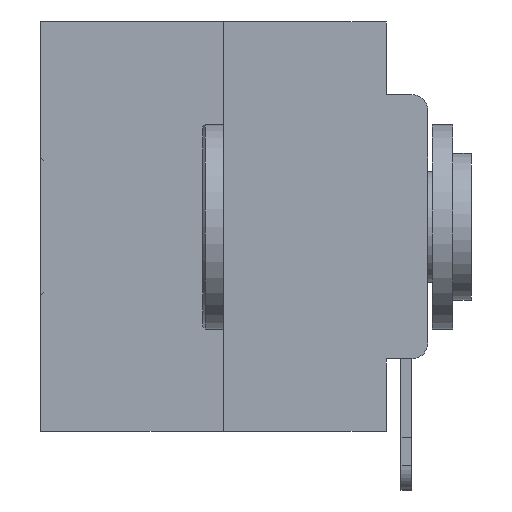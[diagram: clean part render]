
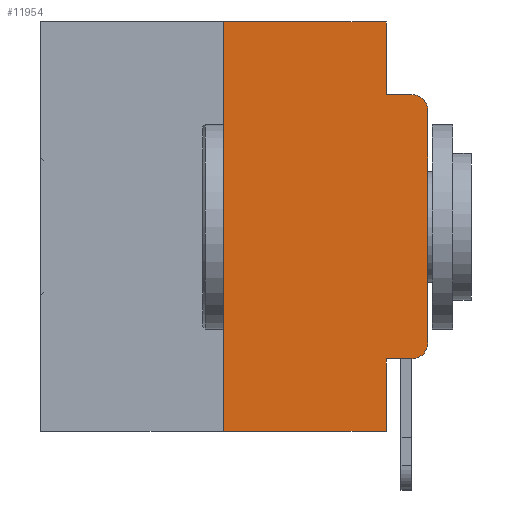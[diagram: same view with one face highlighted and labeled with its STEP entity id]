
A CAD part, left-side view. The second image highlights one B-rep face of the part: STEP entity #11954.
In plain terms, the highlighted planar face has unit normal (-1, 0, 0).
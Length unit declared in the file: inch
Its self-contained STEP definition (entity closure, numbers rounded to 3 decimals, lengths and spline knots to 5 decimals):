
#270 = VERTEX_POINT ( 'NONE', #3833 ) ;
#324 = VECTOR ( 'NONE', #23057, 39.37008 ) ;
#1065 = ORIENTED_EDGE ( 'NONE', *, *, #15553, .F. ) ;
#1364 = VERTEX_POINT ( 'NONE', #24609 ) ;
#1551 = DIRECTION ( 'NONE',  ( 0., -1., 0. ) ) ;
#1678 = CARTESIAN_POINT ( 'NONE',  ( 0., 0.051, -0.4115 ) ) ;
#2303 = VERTEX_POINT ( 'NONE', #25746 ) ;
#2864 = DIRECTION ( 'NONE',  ( -1., 0., 0. ) ) ;
#3169 = ORIENTED_EDGE ( 'NONE', *, *, #7215, .T. ) ;
#3351 = CARTESIAN_POINT ( 'NONE',  ( 0., 0.051, -0.0885 ) ) ;
#3833 = CARTESIAN_POINT ( 'NONE',  ( 0., 0.051, -0.4115 ) ) ;
#3913 = CARTESIAN_POINT ( 'NONE',  ( 0., 0., -0.3915 ) ) ;
#4246 = LINE ( 'NONE', #1678, #11834 ) ;
#4282 = CARTESIAN_POINT ( 'NONE',  ( 0., 0.473, -0.5 ) ) ;
#4827 = DIRECTION ( 'NONE',  ( 0., 0., -1. ) ) ;
#4832 = VECTOR ( 'NONE', #1551, 39.37008 ) ;
#7215 = EDGE_CURVE ( 'NONE', #31424, #12259, #27190, .T. ) ;
#8551 = EDGE_CURVE ( 'NONE', #28924, #19946, #29619, .T. ) ;
#8594 = VECTOR ( 'NONE', #22149, 39.37008 ) ;
#8623 = CARTESIAN_POINT ( 'NONE',  ( 0., 0., -0.1085 ) ) ;
#9428 = LINE ( 'NONE', #31160, #8594 ) ;
#9579 = CARTESIAN_POINT ( 'NONE',  ( 0., 0.02, -0.3915 ) ) ;
#11570 = ORIENTED_EDGE ( 'NONE', *, *, #25066, .F. ) ;
#11834 = VECTOR ( 'NONE', #19168, 39.37008 ) ;
#11904 = VECTOR ( 'NONE', #29697, 39.37008 ) ;
#11954 = ADVANCED_FACE ( 'NONE', ( #16748 ), #31044, .F. ) ;
#12088 = DIRECTION ( 'NONE',  ( 0., 0., -1. ) ) ;
#12253 = VERTEX_POINT ( 'NONE', #23450 ) ;
#12259 = VERTEX_POINT ( 'NONE', #3913 ) ;
#12339 = EDGE_CURVE ( 'NONE', #270, #31424, #4246, .T. ) ;
#12411 = DIRECTION ( 'NONE',  ( 0., 0., -1. ) ) ;
#13102 = CIRCLE ( 'NONE', #13474, 0.02 ) ;
#13474 = AXIS2_PLACEMENT_3D ( 'NONE', #17809, #2864, #20239 ) ;
#15224 = CARTESIAN_POINT ( 'NONE',  ( 0., 0.25, -0.5 ) ) ;
#15553 = EDGE_CURVE ( 'NONE', #270, #12253, #21610, .T. ) ;
#15741 = CARTESIAN_POINT ( 'NONE',  ( 0., 0., 0. ) ) ;
#15785 = EDGE_LOOP ( 'NONE', ( #17207, #23565, #11570, #17952, #18705, #24981, #20217, #1065, #21745, #3169 ) ) ;
#16651 = CARTESIAN_POINT ( 'NONE',  ( 0., 0.473, 0. ) ) ;
#16748 = FACE_OUTER_BOUND ( 'NONE', #15785, .T. ) ;
#17147 = EDGE_CURVE ( 'NONE', #26517, #28924, #9428, .T. ) ;
#17187 = CARTESIAN_POINT ( 'NONE',  ( 0., 0.473, 0. ) ) ;
#17207 = ORIENTED_EDGE ( 'NONE', *, *, #31098, .T. ) ;
#17559 = EDGE_CURVE ( 'NONE', #26517, #12253, #26884, .T. ) ;
#17809 = CARTESIAN_POINT ( 'NONE',  ( 0., 0.02, -0.1085 ) ) ;
#17952 = ORIENTED_EDGE ( 'NONE', *, *, #21983, .F. ) ;
#18024 = VERTEX_POINT ( 'NONE', #8623 ) ;
#18705 = ORIENTED_EDGE ( 'NONE', *, *, #8551, .F. ) ;
#19105 = DIRECTION ( 'NONE',  ( 0., -1., 0. ) ) ;
#19168 = DIRECTION ( 'NONE',  ( 0., -1., 0. ) ) ;
#19599 = DIRECTION ( 'NONE',  ( 1., 0., 0. ) ) ;
#19946 = VERTEX_POINT ( 'NONE', #25311 ) ;
#20047 = DIRECTION ( 'NONE',  ( 0., 0., -1. ) ) ;
#20217 = ORIENTED_EDGE ( 'NONE', *, *, #17559, .T. ) ;
#20239 = DIRECTION ( 'NONE',  ( 0., 0., -1. ) ) ;
#20328 = LINE ( 'NONE', #3351, #324 ) ;
#20421 = LINE ( 'NONE', #22462, #25844 ) ;
#21490 = CARTESIAN_POINT ( 'NONE',  ( 0., 0.02, -0.4115 ) ) ;
#21610 = LINE ( 'NONE', #26538, #27677 ) ;
#21745 = ORIENTED_EDGE ( 'NONE', *, *, #12339, .T. ) ;
#21983 = EDGE_CURVE ( 'NONE', #19946, #2303, #20421, .T. ) ;
#22149 = DIRECTION ( 'NONE',  ( 0., 0., 1. ) ) ;
#22462 = CARTESIAN_POINT ( 'NONE',  ( 0., 0.051, 0. ) ) ;
#23057 = DIRECTION ( 'NONE',  ( 0., -1., 0. ) ) ;
#23450 = CARTESIAN_POINT ( 'NONE',  ( 0., 0.051, -0.5 ) ) ;
#23565 = ORIENTED_EDGE ( 'NONE', *, *, #26559, .T. ) ;
#23865 = AXIS2_PLACEMENT_3D ( 'NONE', #9579, #26249, #12088 ) ;
#24589 = LINE ( 'NONE', #15741, #11904 ) ;
#24609 = CARTESIAN_POINT ( 'NONE',  ( 0., 0.02, -0.0885 ) ) ;
#24981 = ORIENTED_EDGE ( 'NONE', *, *, #17147, .F. ) ;
#25066 = EDGE_CURVE ( 'NONE', #2303, #1364, #20328, .T. ) ;
#25311 = CARTESIAN_POINT ( 'NONE',  ( 0., 0.051, 0. ) ) ;
#25746 = CARTESIAN_POINT ( 'NONE',  ( 0., 0.051, -0.0885 ) ) ;
#25844 = VECTOR ( 'NONE', #20047, 39.37008 ) ;
#26249 = DIRECTION ( 'NONE',  ( -1., 0., 0. ) ) ;
#26517 = VERTEX_POINT ( 'NONE', #15224 ) ;
#26538 = CARTESIAN_POINT ( 'NONE',  ( 0., 0.051, 0. ) ) ;
#26559 = EDGE_CURVE ( 'NONE', #18024, #1364, #13102, .T. ) ;
#26884 = LINE ( 'NONE', #4282, #27595 ) ;
#27190 = CIRCLE ( 'NONE', #23865, 0.02 ) ;
#27595 = VECTOR ( 'NONE', #19105, 39.37008 ) ;
#27677 = VECTOR ( 'NONE', #12411, 39.37008 ) ;
#28924 = VERTEX_POINT ( 'NONE', #31359 ) ;
#29619 = LINE ( 'NONE', #16651, #4832 ) ;
#29697 = DIRECTION ( 'NONE',  ( 0., 0., 1. ) ) ;
#31044 = PLANE ( 'NONE',  #31157 ) ;
#31098 = EDGE_CURVE ( 'NONE', #12259, #18024, #24589, .T. ) ;
#31157 = AXIS2_PLACEMENT_3D ( 'NONE', #17187, #19599, #4827 ) ;
#31160 = CARTESIAN_POINT ( 'NONE',  ( 0., 0.25, 0. ) ) ;
#31359 = CARTESIAN_POINT ( 'NONE',  ( 0., 0.25, 0. ) ) ;
#31424 = VERTEX_POINT ( 'NONE', #21490 ) ;
